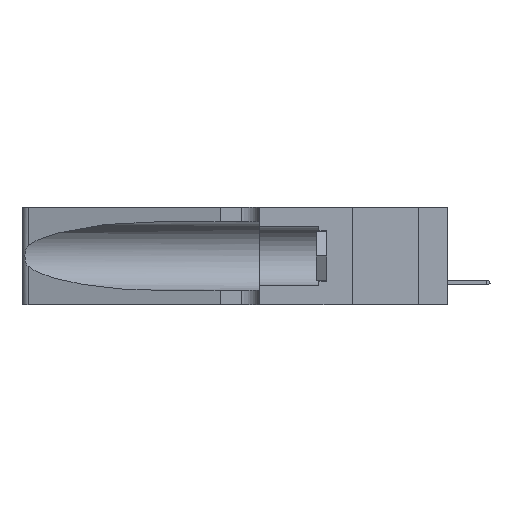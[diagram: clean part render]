
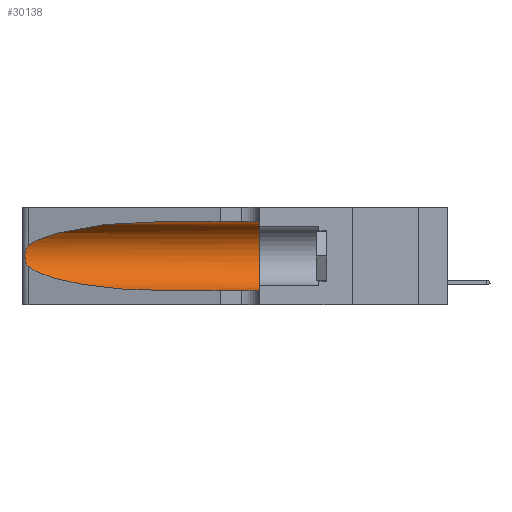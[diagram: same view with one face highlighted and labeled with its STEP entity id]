
A CAD part, left-side view. The second image highlights one B-rep face of the part: STEP entity #30138.
In plain terms, the highlighted cylindrical face has radius 3.308 mm (diameter 6.617 mm), a partial arc.
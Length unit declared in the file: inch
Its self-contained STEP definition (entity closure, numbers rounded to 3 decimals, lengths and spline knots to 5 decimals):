
#1794 = VERTEX_POINT ( 'NONE', #26986 ) ;
#2441 = CARTESIAN_POINT ( 'NONE',  ( 0.26018, 1.23835, 0.19895 ) ) ;
#3144 = CARTESIAN_POINT ( 'NONE',  ( 0.18966, 0.96281, 0.05475 ) ) ;
#3423 = DIRECTION ( 'NONE',  ( 0., -1., 0. ) ) ;
#4282 = AXIS2_PLACEMENT_3D ( 'NONE', #19734, #35860, #32133 ) ;
#4460 = EDGE_CURVE ( 'NONE', #1794, #21478, #9588, .T. ) ;
#7568 = CYLINDRICAL_SURFACE ( 'NONE', #23077, 0.13025 ) ;
#7751 = CARTESIAN_POINT ( 'NONE',  ( 0.1305, 0.35, 0.31525 ) ) ;
#8859 = ORIENTED_EDGE ( 'NONE', *, *, #30158, .F. ) ;
#9091 = CARTESIAN_POINT ( 'NONE',  ( 0.25487, 1.22718, 0.14631 ) ) ;
#9588 = LINE ( 'NONE', #34324, #29617 ) ;
#9944 = CARTESIAN_POINT ( 'NONE',  ( 0.18966, 0.96281, 0.31525 ) ) ;
#10776 = CARTESIAN_POINT ( 'NONE',  ( 0.25487, 1.22718, 0.22369 ) ) ;
#13674 = CARTESIAN_POINT ( 'NONE',  ( 0.26017, 1.23833, 0.17102 ) ) ;
#17305 = ORIENTED_EDGE ( 'NONE', *, *, #41361, .T. ) ;
#17841 = B_SPLINE_CURVE_WITH_KNOTS ( 'NONE', 3,
 ( #38189, #37650, #22193, #18405, #33992, #2441, #30473, #34358, #13674, #50042, #45811, #46008, #42038, #49677 ),
 .UNSPECIFIED., .F., .F.,
 ( 4, 2, 2, 2, 2, 2, 4 ),
 ( 0., 0.00027, 0.00053, 0.00107, 0.0016, 0.00187, 0.00214 ),
 .UNSPECIFIED. ) ;
#18288 = ORIENTED_EDGE ( 'NONE', *, *, #30422, .F. ) ;
#18405 = CARTESIAN_POINT ( 'NONE',  ( 0.25787, 1.23484, 0.2124 ) ) ;
#18526 =( BOUNDED_CURVE ( )  B_SPLINE_CURVE ( 3, ( #26242, #9944, #35731, #24060 ),
 .UNSPECIFIED., .F., .F. ) 
 B_SPLINE_CURVE_WITH_KNOTS ( ( 4, 4 ),
 ( 1.5708, 2.84003 ),
 .UNSPECIFIED. ) 
 CURVE ( )  GEOMETRIC_REPRESENTATION_ITEM ( )  RATIONAL_B_SPLINE_CURVE ( ( 1., 0.87, 0.87, 1. ) ) 
 REPRESENTATION_ITEM ( '' )  );
#19395 = CARTESIAN_POINT ( 'NONE',  ( 0.1305, 1.61858, 0.31525 ) ) ;
#19734 = CARTESIAN_POINT ( 'NONE',  ( 0.1305, 0.35, 0.185 ) ) ;
#19819 = VERTEX_POINT ( 'NONE', #44453 ) ;
#21478 = VERTEX_POINT ( 'NONE', #37659 ) ;
#22193 = CARTESIAN_POINT ( 'NONE',  ( 0.25639, 1.23184, 0.21858 ) ) ;
#22510 = DIRECTION ( 'NONE',  ( 0., -1., 0. ) ) ;
#22697 = CARTESIAN_POINT ( 'NONE',  ( 0.1305, 0.72297, 0.05475 ) ) ;
#23077 = AXIS2_PLACEMENT_3D ( 'NONE', #27204, #3423, #31286 ) ;
#24060 = CARTESIAN_POINT ( 'NONE',  ( 0.25487, 1.22718, 0.22369 ) ) ;
#26242 = CARTESIAN_POINT ( 'NONE',  ( 0.1305, 0.72297, 0.31525 ) ) ;
#26986 = CARTESIAN_POINT ( 'NONE',  ( 0.1305, 0.72297, 0.05475 ) ) ;
#27021 = ORIENTED_EDGE ( 'NONE', *, *, #4460, .T. ) ;
#27204 = CARTESIAN_POINT ( 'NONE',  ( 0.1305, 1.61858, 0.185 ) ) ;
#28092 = EDGE_LOOP ( 'NONE', ( #17305, #30140, #37630, #27021, #18288, #8859 ) ) ;
#29617 = VECTOR ( 'NONE', #22510, 39.37008 ) ;
#30138 = ADVANCED_FACE ( 'NONE', ( #35200 ), #7568, .F. ) ;
#30140 = ORIENTED_EDGE ( 'NONE', *, *, #40386, .T. ) ;
#30158 = EDGE_CURVE ( 'NONE', #19819, #43333, #34528, .T. ) ;
#30422 = EDGE_CURVE ( 'NONE', #43333, #21478, #48793, .T. ) ;
#30473 = CARTESIAN_POINT ( 'NONE',  ( 0.26075, 1.23896, 0.19203 ) ) ;
#31286 = DIRECTION ( 'NONE',  ( 0., 0., -1. ) ) ;
#32133 = DIRECTION ( 'NONE',  ( 0., 0., 1. ) ) ;
#32578 =( BOUNDED_CURVE ( )  B_SPLINE_CURVE ( 3, ( #51141, #32836, #3144, #22697 ),
 .UNSPECIFIED., .F., .T. ) 
 B_SPLINE_CURVE_WITH_KNOTS ( ( 4, 4 ),
 ( 3.44316, 4.71239 ),
 .UNSPECIFIED. ) 
 CURVE ( )  GEOMETRIC_REPRESENTATION_ITEM ( )  RATIONAL_B_SPLINE_CURVE ( ( 1., 0.87, 0.87, 1. ) ) 
 REPRESENTATION_ITEM ( '' )  );
#32836 = CARTESIAN_POINT ( 'NONE',  ( 0.2373, 1.15595, 0.08982 ) ) ;
#33458 = VERTEX_POINT ( 'NONE', #9091 ) ;
#33992 = CARTESIAN_POINT ( 'NONE',  ( 0.25854, 1.2359, 0.20912 ) ) ;
#34324 = CARTESIAN_POINT ( 'NONE',  ( 0.1305, 1.61858, 0.05475 ) ) ;
#34358 = CARTESIAN_POINT ( 'NONE',  ( 0.26075, 1.23896, 0.178 ) ) ;
#34528 = LINE ( 'NONE', #19395, #35797 ) ;
#35200 = FACE_OUTER_BOUND ( 'NONE', #28092, .T. ) ;
#35731 = CARTESIAN_POINT ( 'NONE',  ( 0.2373, 1.15595, 0.28018 ) ) ;
#35797 = VECTOR ( 'NONE', #43854, 39.37008 ) ;
#35860 = DIRECTION ( 'NONE',  ( 0., 1., 0. ) ) ;
#37630 = ORIENTED_EDGE ( 'NONE', *, *, #39701, .T. ) ;
#37650 = CARTESIAN_POINT ( 'NONE',  ( 0.25555, 1.22994, 0.2215 ) ) ;
#37659 = CARTESIAN_POINT ( 'NONE',  ( 0.1305, 0.35, 0.05475 ) ) ;
#38189 = CARTESIAN_POINT ( 'NONE',  ( 0.25487, 1.22718, 0.22369 ) ) ;
#39701 = EDGE_CURVE ( 'NONE', #33458, #1794, #32578, .T. ) ;
#40386 = EDGE_CURVE ( 'NONE', #50348, #33458, #17841, .T. ) ;
#41361 = EDGE_CURVE ( 'NONE', #19819, #50348, #18526, .T. ) ;
#42038 = CARTESIAN_POINT ( 'NONE',  ( 0.25555, 1.22993, 0.14849 ) ) ;
#43333 = VERTEX_POINT ( 'NONE', #7751 ) ;
#43854 = DIRECTION ( 'NONE',  ( 0., -1., 0. ) ) ;
#44453 = CARTESIAN_POINT ( 'NONE',  ( 0.1305, 0.72297, 0.31525 ) ) ;
#45811 = CARTESIAN_POINT ( 'NONE',  ( 0.25789, 1.23486, 0.15765 ) ) ;
#46008 = CARTESIAN_POINT ( 'NONE',  ( 0.25639, 1.23186, 0.15144 ) ) ;
#48793 = CIRCLE ( 'NONE', #4282, 0.13025 ) ;
#49677 = CARTESIAN_POINT ( 'NONE',  ( 0.25487, 1.22718, 0.14631 ) ) ;
#50042 = CARTESIAN_POINT ( 'NONE',  ( 0.25856, 1.23593, 0.16098 ) ) ;
#50348 = VERTEX_POINT ( 'NONE', #10776 ) ;
#51141 = CARTESIAN_POINT ( 'NONE',  ( 0.25487, 1.22718, 0.14631 ) ) ;
